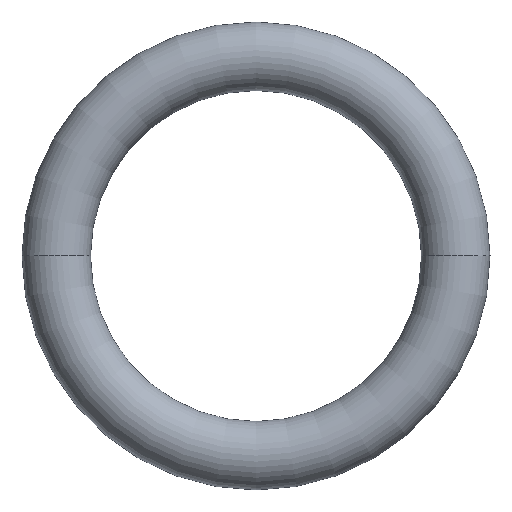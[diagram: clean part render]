
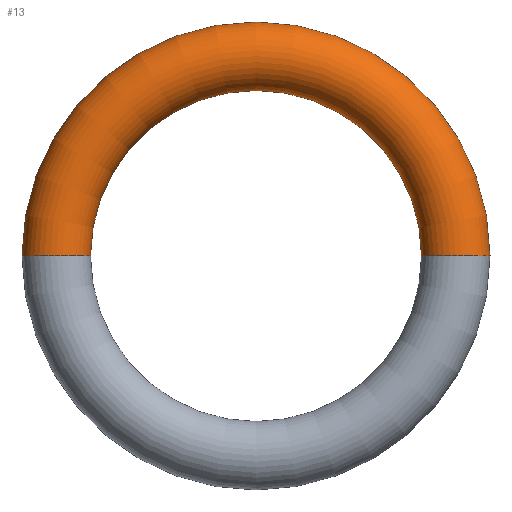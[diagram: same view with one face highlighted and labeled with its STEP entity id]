
A CAD part, top view. The second image highlights one B-rep face of the part: STEP entity #13.
In plain terms, the highlighted toroidal (fillet/blend) face has major radius 4.445 mm and minor radius 0.762 mm.
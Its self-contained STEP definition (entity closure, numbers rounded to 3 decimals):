
#1 = AXIS2_PLACEMENT_3D ( 'NONE', #71, #113, #150 ) ;
#2 = CARTESIAN_POINT ( 'NONE',  ( 0., 0., 0. ) ) ;
#4 = TOROIDAL_SURFACE ( 'NONE', #90, 4.445, 0.762 ) ;
#8 = CIRCLE ( 'NONE', #1, 0.762 ) ;
#9 = VERTEX_POINT ( 'NONE', #81 ) ;
#11 = CIRCLE ( 'NONE', #96, 0.762 ) ;
#13 = ADVANCED_FACE ( 'NONE', ( #23 ), #4, .T. ) ;
#23 = FACE_OUTER_BOUND ( 'NONE', #59, .T. ) ;
#24 = CIRCLE ( 'NONE', #146, 3.683 ) ;
#28 = VERTEX_POINT ( 'NONE', #119 ) ;
#33 = VERTEX_POINT ( 'NONE', #76 ) ;
#38 = VERTEX_POINT ( 'NONE', #49 ) ;
#45 = DIRECTION ( 'NONE',  ( 0., 0., -1. ) ) ;
#49 = CARTESIAN_POINT ( 'NONE',  ( -3.683, 0., 0. ) ) ;
#50 = ORIENTED_EDGE ( 'NONE', *, *, #123, .F. ) ;
#54 = ORIENTED_EDGE ( 'NONE', *, *, #92, .F. ) ;
#56 = ORIENTED_EDGE ( 'NONE', *, *, #91, .T. ) ;
#57 = ORIENTED_EDGE ( 'NONE', *, *, #120, .T. ) ;
#59 = EDGE_LOOP ( 'NONE', ( #50, #54, #57, #56 ) ) ;
#61 = DIRECTION ( 'NONE',  ( 0., 0., -1. ) ) ;
#63 = CIRCLE ( 'NONE', #143, 5.207 ) ;
#64 = CARTESIAN_POINT ( 'NONE',  ( 0., 0., 0. ) ) ;
#67 = CARTESIAN_POINT ( 'NONE',  ( 0., 0., 0. ) ) ;
#69 = DIRECTION ( 'NONE',  ( -1., 0., 0. ) ) ;
#71 = CARTESIAN_POINT ( 'NONE',  ( -4.445, 0., 0. ) ) ;
#74 = CARTESIAN_POINT ( 'NONE',  ( 4.445, 0., 0. ) ) ;
#76 = CARTESIAN_POINT ( 'NONE',  ( -5.207, 0., 0. ) ) ;
#81 = CARTESIAN_POINT ( 'NONE',  ( 5.207, 0., 0. ) ) ;
#90 = AXIS2_PLACEMENT_3D ( 'NONE', #2, #61, #124 ) ;
#91 = EDGE_CURVE ( 'NONE', #28, #9, #11, .T. ) ;
#92 = EDGE_CURVE ( 'NONE', #38, #33, #8, .T. ) ;
#96 = AXIS2_PLACEMENT_3D ( 'NONE', #74, #125, #118 ) ;
#113 = DIRECTION ( 'NONE',  ( 0., -1., 0. ) ) ;
#118 = DIRECTION ( 'NONE',  ( -1., 0., 0. ) ) ;
#119 = CARTESIAN_POINT ( 'NONE',  ( 3.683, 0., 0. ) ) ;
#120 = EDGE_CURVE ( 'NONE', #38, #28, #24, .T. ) ;
#123 = EDGE_CURVE ( 'NONE', #33, #9, #63, .T. ) ;
#124 = DIRECTION ( 'NONE',  ( -1., 0., 0. ) ) ;
#125 = DIRECTION ( 'NONE',  ( 0., 1., 0. ) ) ;
#134 = DIRECTION ( 'NONE',  ( 0., 0., -1. ) ) ;
#143 = AXIS2_PLACEMENT_3D ( 'NONE', #67, #134, #69 ) ;
#146 = AXIS2_PLACEMENT_3D ( 'NONE', #64, #45, #154 ) ;
#150 = DIRECTION ( 'NONE',  ( 0., 0., -1. ) ) ;
#154 = DIRECTION ( 'NONE',  ( -1., 0., 0. ) ) ;
